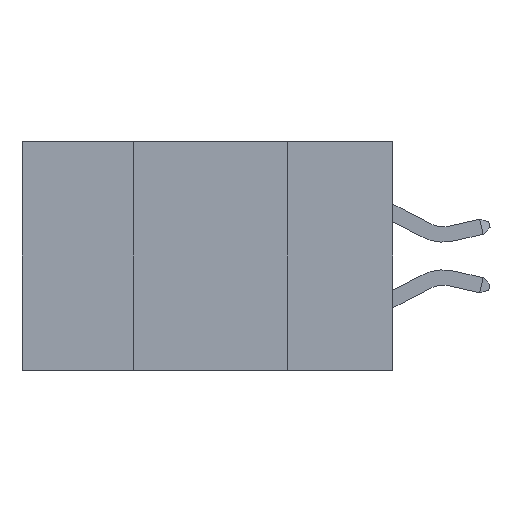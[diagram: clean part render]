
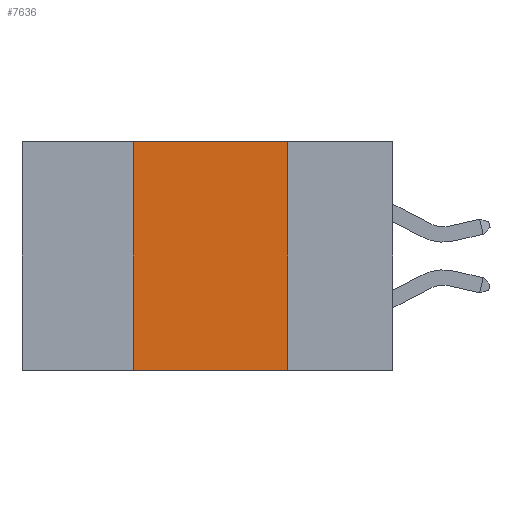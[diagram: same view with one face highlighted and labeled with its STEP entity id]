
A CAD part, left-side view. The second image highlights one B-rep face of the part: STEP entity #7636.
In plain terms, the highlighted planar face has unit normal (-1, 0, 0).
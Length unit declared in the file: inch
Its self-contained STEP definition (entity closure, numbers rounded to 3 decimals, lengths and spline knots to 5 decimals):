
#1176 = LINE ( 'NONE', #36480, #8103 ) ;
#1324 = DIRECTION ( 'NONE',  ( 0., 0., -1. ) ) ;
#2820 = CARTESIAN_POINT ( 'NONE',  ( 0., 0.42, 0. ) ) ;
#2830 = DIRECTION ( 'NONE',  ( 0., -1., 0. ) ) ;
#3885 = FACE_OUTER_BOUND ( 'NONE', #33542, .T. ) ;
#4662 = DIRECTION ( 'NONE',  ( 1., 0., 0. ) ) ;
#5003 = VERTEX_POINT ( 'NONE', #34263 ) ;
#6561 = CARTESIAN_POINT ( 'NONE',  ( 0., 0.6, -0.37 ) ) ;
#6588 = ORIENTED_EDGE ( 'NONE', *, *, #22433, .F. ) ;
#7636 = ADVANCED_FACE ( 'NONE', ( #3885 ), #13142, .F. ) ;
#8103 = VECTOR ( 'NONE', #15378, 39.37008 ) ;
#9845 = LINE ( 'NONE', #30406, #33364 ) ;
#10389 = CARTESIAN_POINT ( 'NONE',  ( 0., 0.6, 0. ) ) ;
#13142 = PLANE ( 'NONE',  #30195 ) ;
#14012 = VECTOR ( 'NONE', #2830, 39.37008 ) ;
#14999 = EDGE_CURVE ( 'NONE', #36158, #5003, #36544, .T. ) ;
#15179 = ORIENTED_EDGE ( 'NONE', *, *, #26651, .F. ) ;
#15378 = DIRECTION ( 'NONE',  ( 0., 0., -1. ) ) ;
#20954 = DIRECTION ( 'NONE',  ( 0., 0., 1. ) ) ;
#21235 = CARTESIAN_POINT ( 'NONE',  ( 0., 0.17, 0. ) ) ;
#22433 = EDGE_CURVE ( 'NONE', #5003, #30839, #9845, .T. ) ;
#24083 = VERTEX_POINT ( 'NONE', #31642 ) ;
#26651 = EDGE_CURVE ( 'NONE', #30839, #24083, #1176, .T. ) ;
#30195 = AXIS2_PLACEMENT_3D ( 'NONE', #10389, #4662, #1324 ) ;
#30196 = DIRECTION ( 'NONE',  ( 0., -1., 0. ) ) ;
#30320 = ORIENTED_EDGE ( 'NONE', *, *, #33145, .T. ) ;
#30406 = CARTESIAN_POINT ( 'NONE',  ( 0., 0.6, 0. ) ) ;
#30470 = CARTESIAN_POINT ( 'NONE',  ( 0., 0.42, -0.37 ) ) ;
#30839 = VERTEX_POINT ( 'NONE', #21235 ) ;
#31642 = CARTESIAN_POINT ( 'NONE',  ( 0., 0.17, -0.37 ) ) ;
#31807 = VECTOR ( 'NONE', #20954, 39.37008 ) ;
#33145 = EDGE_CURVE ( 'NONE', #36158, #24083, #33616, .T. ) ;
#33364 = VECTOR ( 'NONE', #30196, 39.37008 ) ;
#33542 = EDGE_LOOP ( 'NONE', ( #15179, #6588, #34711, #30320 ) ) ;
#33616 = LINE ( 'NONE', #6561, #14012 ) ;
#34263 = CARTESIAN_POINT ( 'NONE',  ( 0., 0.42, 0. ) ) ;
#34711 = ORIENTED_EDGE ( 'NONE', *, *, #14999, .F. ) ;
#36158 = VERTEX_POINT ( 'NONE', #30470 ) ;
#36480 = CARTESIAN_POINT ( 'NONE',  ( 0., 0.17, 0. ) ) ;
#36544 = LINE ( 'NONE', #2820, #31807 ) ;
